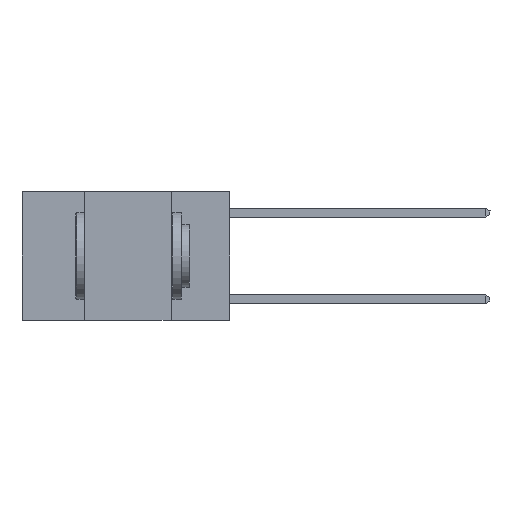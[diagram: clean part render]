
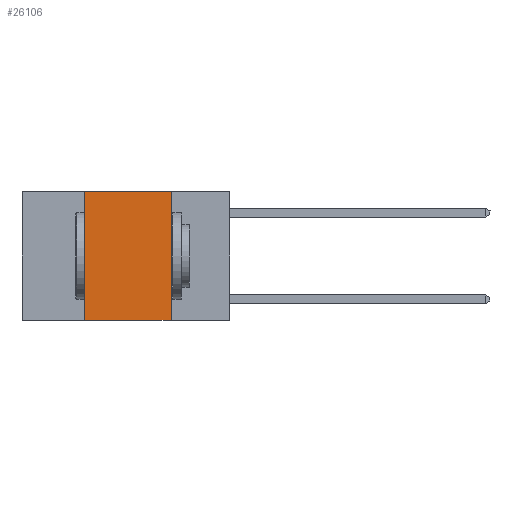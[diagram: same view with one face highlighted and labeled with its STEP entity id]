
A CAD part, left-side view. The second image highlights one B-rep face of the part: STEP entity #26106.
In plain terms, the highlighted planar face has unit normal (-1, 0, 0).
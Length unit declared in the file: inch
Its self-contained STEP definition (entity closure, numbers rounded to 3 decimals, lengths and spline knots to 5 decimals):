
#1160 = ORIENTED_EDGE ( 'NONE', *, *, #7340, .F. ) ;
#1322 = VERTEX_POINT ( 'NONE', #8613 ) ;
#3381 = ORIENTED_EDGE ( 'NONE', *, *, #5257, .T. ) ;
#4017 = VECTOR ( 'NONE', #19646, 39.37008 ) ;
#4148 = CARTESIAN_POINT ( 'NONE',  ( 0., 0.42, 0. ) ) ;
#4990 = LINE ( 'NONE', #9824, #4017 ) ;
#5257 = EDGE_CURVE ( 'NONE', #11051, #1322, #30624, .T. ) ;
#6824 = DIRECTION ( 'NONE',  ( 0., 0., -1. ) ) ;
#7340 = EDGE_CURVE ( 'NONE', #19445, #1322, #4990, .T. ) ;
#8437 = LINE ( 'NONE', #13412, #12500 ) ;
#8604 = CARTESIAN_POINT ( 'NONE',  ( 0., 0.6, -0.37 ) ) ;
#8613 = CARTESIAN_POINT ( 'NONE',  ( 0., 0.17, -0.37 ) ) ;
#9824 = CARTESIAN_POINT ( 'NONE',  ( 0., 0.17, 0. ) ) ;
#10454 = CARTESIAN_POINT ( 'NONE',  ( 0., 0.42, 0. ) ) ;
#11051 = VERTEX_POINT ( 'NONE', #17260 ) ;
#12050 = ORIENTED_EDGE ( 'NONE', *, *, #22442, .F. ) ;
#12500 = VECTOR ( 'NONE', #23252, 39.37008 ) ;
#13412 = CARTESIAN_POINT ( 'NONE',  ( 0., 0.6, 0. ) ) ;
#14270 = AXIS2_PLACEMENT_3D ( 'NONE', #23595, #28540, #6824 ) ;
#15253 = VERTEX_POINT ( 'NONE', #4148 ) ;
#16951 = CARTESIAN_POINT ( 'NONE',  ( 0., 0.17, 0. ) ) ;
#17260 = CARTESIAN_POINT ( 'NONE',  ( 0., 0.42, -0.37 ) ) ;
#17408 = EDGE_LOOP ( 'NONE', ( #1160, #30442, #12050, #3381 ) ) ;
#17485 = EDGE_CURVE ( 'NONE', #15253, #19445, #8437, .T. ) ;
#17776 = VECTOR ( 'NONE', #30216, 39.37008 ) ;
#18010 = LINE ( 'NONE', #10454, #17776 ) ;
#19366 = VECTOR ( 'NONE', #27891, 39.37008 ) ;
#19445 = VERTEX_POINT ( 'NONE', #16951 ) ;
#19646 = DIRECTION ( 'NONE',  ( 0., 0., -1. ) ) ;
#21030 = FACE_OUTER_BOUND ( 'NONE', #17408, .T. ) ;
#21180 = PLANE ( 'NONE',  #14270 ) ;
#22442 = EDGE_CURVE ( 'NONE', #11051, #15253, #18010, .T. ) ;
#23252 = DIRECTION ( 'NONE',  ( 0., -1., 0. ) ) ;
#23595 = CARTESIAN_POINT ( 'NONE',  ( 0., 0.6, 0. ) ) ;
#26106 = ADVANCED_FACE ( 'NONE', ( #21030 ), #21180, .F. ) ;
#27891 = DIRECTION ( 'NONE',  ( 0., -1., 0. ) ) ;
#28540 = DIRECTION ( 'NONE',  ( 1., 0., 0. ) ) ;
#30216 = DIRECTION ( 'NONE',  ( 0., 0., 1. ) ) ;
#30442 = ORIENTED_EDGE ( 'NONE', *, *, #17485, .F. ) ;
#30624 = LINE ( 'NONE', #8604, #19366 ) ;
